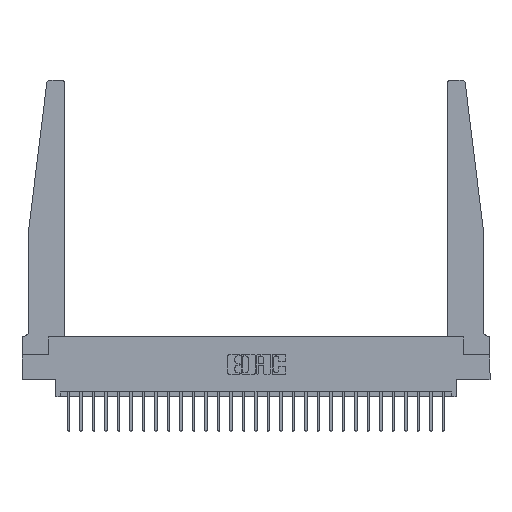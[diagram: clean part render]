
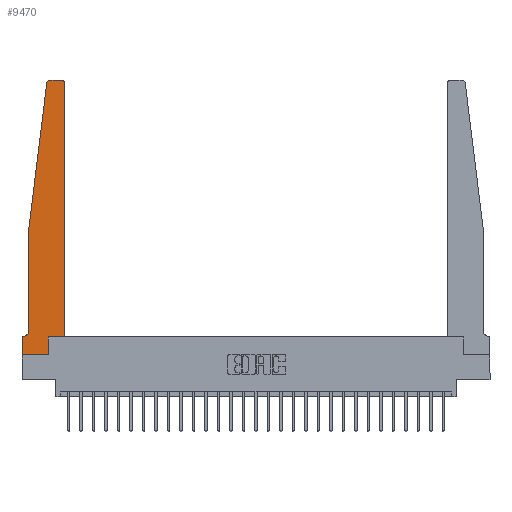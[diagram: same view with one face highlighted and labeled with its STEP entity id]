
A CAD part, top view. The second image highlights one B-rep face of the part: STEP entity #9470.
In plain terms, the highlighted planar face has unit normal (0, 0, 1).
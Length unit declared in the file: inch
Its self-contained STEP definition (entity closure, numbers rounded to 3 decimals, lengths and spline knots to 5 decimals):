
#111 = VERTEX_POINT ( 'NONE', #14592 ) ;
#221 = EDGE_CURVE ( 'NONE', #11357, #2797, #7711, .T. ) ;
#280 = LINE ( 'NONE', #23673, #10578 ) ;
#2040 = CARTESIAN_POINT ( 'NONE',  ( 0.015, 0.1875, 0.37 ) ) ;
#2069 = CARTESIAN_POINT ( 'NONE',  ( 0.425, 0.18, 0.37 ) ) ;
#2569 = ORIENTED_EDGE ( 'NONE', *, *, #17596, .T. ) ;
#2797 = VERTEX_POINT ( 'NONE', #4165 ) ;
#2883 = CARTESIAN_POINT ( 'NONE',  ( 0., 0., 0.37 ) ) ;
#3174 = DIRECTION ( 'NONE',  ( -0.122, -0.992, 0. ) ) ;
#3712 = CARTESIAN_POINT ( 'NONE',  ( 0.2605, 0.18, 0.37 ) ) ;
#3893 = EDGE_CURVE ( 'NONE', #19799, #4411, #19033, .T. ) ;
#4141 = DIRECTION ( 'NONE',  ( 1., 0., 0. ) ) ;
#4165 = CARTESIAN_POINT ( 'NONE',  ( 0., 0., 0.37 ) ) ;
#4411 = VERTEX_POINT ( 'NONE', #3712 ) ;
#4615 = CARTESIAN_POINT ( 'NONE',  ( 0., 0., 0.37 ) ) ;
#4736 = CARTESIAN_POINT ( 'NONE',  ( 0., 0.1875, 0.37 ) ) ;
#4929 = DIRECTION ( 'NONE',  ( 1., 0., 0. ) ) ;
#5170 = CARTESIAN_POINT ( 'NONE',  ( 0.27653, 2.72, 0.37 ) ) ;
#5223 = CARTESIAN_POINT ( 'NONE',  ( 0.065, 1.25, 0.37 ) ) ;
#5352 = LINE ( 'NONE', #15770, #15010 ) ;
#5483 = CARTESIAN_POINT ( 'NONE',  ( 0.425, 2.72, 0.37 ) ) ;
#5676 = ORIENTED_EDGE ( 'NONE', *, *, #12274, .T. ) ;
#5800 = CARTESIAN_POINT ( 'NONE',  ( 0.24675, 2.72367, 0.37 ) ) ;
#6036 = CARTESIAN_POINT ( 'NONE',  ( 0.395, 2.75, 0.37 ) ) ;
#6667 = DIRECTION ( 'NONE',  ( 0., -1., 0. ) ) ;
#6831 = ORIENTED_EDGE ( 'NONE', *, *, #18701, .T. ) ;
#7228 = DIRECTION ( 'NONE',  ( 1., 0., 0. ) ) ;
#7288 = DIRECTION ( 'NONE',  ( 0., -1., 0. ) ) ;
#7426 = LINE ( 'NONE', #10657, #23231 ) ;
#7565 = DIRECTION ( 'NONE',  ( 0., 1., 0. ) ) ;
#7711 = LINE ( 'NONE', #4615, #12566 ) ;
#8064 = VECTOR ( 'NONE', #12185, 39.37008 ) ;
#8595 = LINE ( 'NONE', #20922, #14055 ) ;
#8622 = PLANE ( 'NONE',  #11605 ) ;
#8932 = LINE ( 'NONE', #2069, #24058 ) ;
#9004 = EDGE_CURVE ( 'NONE', #26423, #25578, #12305, .T. ) ;
#9470 = ADVANCED_FACE ( 'NONE', ( #14862 ), #8622, .T. ) ;
#10116 = CARTESIAN_POINT ( 'NONE',  ( 0.2605, 0.18, 0.37 ) ) ;
#10255 = ORIENTED_EDGE ( 'NONE', *, *, #18829, .T. ) ;
#10534 = CIRCLE ( 'NONE', #11642, 0.05 ) ;
#10556 = CARTESIAN_POINT ( 'NONE',  ( 0.015, 0.2375, 0.37 ) ) ;
#10578 = VECTOR ( 'NONE', #3174, 39.37008 ) ;
#10657 = CARTESIAN_POINT ( 'NONE',  ( 0.065, 0.1875, 0.37 ) ) ;
#10686 = DIRECTION ( 'NONE',  ( 0., 0., 1. ) ) ;
#10971 = CARTESIAN_POINT ( 'NONE',  ( 0.065, 0.2375, 0.37 ) ) ;
#11335 = ORIENTED_EDGE ( 'NONE', *, *, #15818, .T. ) ;
#11357 = VERTEX_POINT ( 'NONE', #4736 ) ;
#11605 = AXIS2_PLACEMENT_3D ( 'NONE', #23038, #10686, #25107 ) ;
#11628 = VERTEX_POINT ( 'NONE', #2040 ) ;
#11642 = AXIS2_PLACEMENT_3D ( 'NONE', #10556, #24960, #12614 ) ;
#11795 = CARTESIAN_POINT ( 'NONE',  ( 0.395, 2.72, 0.37 ) ) ;
#12027 = CARTESIAN_POINT ( 'NONE',  ( 0.065, 1.25, 0.37 ) ) ;
#12185 = DIRECTION ( 'NONE',  ( 0., 1., 0. ) ) ;
#12243 = EDGE_CURVE ( 'NONE', #25578, #11628, #10534, .T. ) ;
#12270 = AXIS2_PLACEMENT_3D ( 'NONE', #11795, #26187, #13844 ) ;
#12274 = EDGE_CURVE ( 'NONE', #19041, #111, #8595, .T. ) ;
#12305 = LINE ( 'NONE', #5223, #22627 ) ;
#12566 = VECTOR ( 'NONE', #6667, 39.37008 ) ;
#12579 = VERTEX_POINT ( 'NONE', #5483 ) ;
#12614 = DIRECTION ( 'NONE',  ( -1., 0., 0. ) ) ;
#12836 = EDGE_CURVE ( 'NONE', #4411, #26561, #8932, .T. ) ;
#13183 = ORIENTED_EDGE ( 'NONE', *, *, #19515, .T. ) ;
#13543 = ORIENTED_EDGE ( 'NONE', *, *, #9004, .T. ) ;
#13663 = VECTOR ( 'NONE', #4929, 39.37008 ) ;
#13844 = DIRECTION ( 'NONE',  ( 1., 0., 0. ) ) ;
#14055 = VECTOR ( 'NONE', #14774, 39.37008 ) ;
#14058 = ORIENTED_EDGE ( 'NONE', *, *, #12243, .T. ) ;
#14592 = CARTESIAN_POINT ( 'NONE',  ( 0.27653, 2.75, 0.37 ) ) ;
#14774 = DIRECTION ( 'NONE',  ( -1., 0., 0. ) ) ;
#14862 = FACE_OUTER_BOUND ( 'NONE', #17558, .T. ) ;
#15010 = VECTOR ( 'NONE', #7565, 39.37008 ) ;
#15770 = CARTESIAN_POINT ( 'NONE',  ( 0.425, 0.18, 0.37 ) ) ;
#15818 = EDGE_CURVE ( 'NONE', #11628, #11357, #7426, .T. ) ;
#17225 = ORIENTED_EDGE ( 'NONE', *, *, #221, .T. ) ;
#17239 = CIRCLE ( 'NONE', #12270, 0.03 ) ;
#17558 = EDGE_LOOP ( 'NONE', ( #5676, #6831, #2569, #13543, #14058, #11335, #17225, #26530, #21107, #20203, #10255, #13183 ) ) ;
#17596 = EDGE_CURVE ( 'NONE', #22145, #26423, #280, .T. ) ;
#18701 = EDGE_CURVE ( 'NONE', #111, #22145, #23718, .T. ) ;
#18829 = EDGE_CURVE ( 'NONE', #26561, #12579, #5352, .T. ) ;
#19033 = LINE ( 'NONE', #10116, #8064 ) ;
#19041 = VERTEX_POINT ( 'NONE', #6036 ) ;
#19154 = LINE ( 'NONE', #2883, #13663 ) ;
#19515 = EDGE_CURVE ( 'NONE', #12579, #19041, #17239, .T. ) ;
#19581 = DIRECTION ( 'NONE',  ( 0., 0., 1. ) ) ;
#19799 = VERTEX_POINT ( 'NONE', #23131 ) ;
#19899 = EDGE_CURVE ( 'NONE', #2797, #19799, #19154, .T. ) ;
#20203 = ORIENTED_EDGE ( 'NONE', *, *, #12836, .T. ) ;
#20217 = AXIS2_PLACEMENT_3D ( 'NONE', #5170, #19581, #7228 ) ;
#20922 = CARTESIAN_POINT ( 'NONE',  ( 0.25, 2.75, 0.37 ) ) ;
#21107 = ORIENTED_EDGE ( 'NONE', *, *, #3893, .T. ) ;
#22145 = VERTEX_POINT ( 'NONE', #5800 ) ;
#22627 = VECTOR ( 'NONE', #7288, 39.37008 ) ;
#22999 = DIRECTION ( 'NONE',  ( -1., 0., 0. ) ) ;
#23038 = CARTESIAN_POINT ( 'NONE',  ( 0., 0.1875, 0.37 ) ) ;
#23131 = CARTESIAN_POINT ( 'NONE',  ( 0.2605, 0., 0.37 ) ) ;
#23231 = VECTOR ( 'NONE', #22999, 39.37008 ) ;
#23673 = CARTESIAN_POINT ( 'NONE',  ( 0.065, 1.25, 0.37 ) ) ;
#23718 = CIRCLE ( 'NONE', #20217, 0.03 ) ;
#24058 = VECTOR ( 'NONE', #4141, 39.37008 ) ;
#24728 = CARTESIAN_POINT ( 'NONE',  ( 0.425, 0.18, 0.37 ) ) ;
#24960 = DIRECTION ( 'NONE',  ( 0., 0., -1. ) ) ;
#25107 = DIRECTION ( 'NONE',  ( 1., 0., 0. ) ) ;
#25578 = VERTEX_POINT ( 'NONE', #10971 ) ;
#26187 = DIRECTION ( 'NONE',  ( 0., 0., 1. ) ) ;
#26423 = VERTEX_POINT ( 'NONE', #12027 ) ;
#26530 = ORIENTED_EDGE ( 'NONE', *, *, #19899, .T. ) ;
#26561 = VERTEX_POINT ( 'NONE', #24728 ) ;
